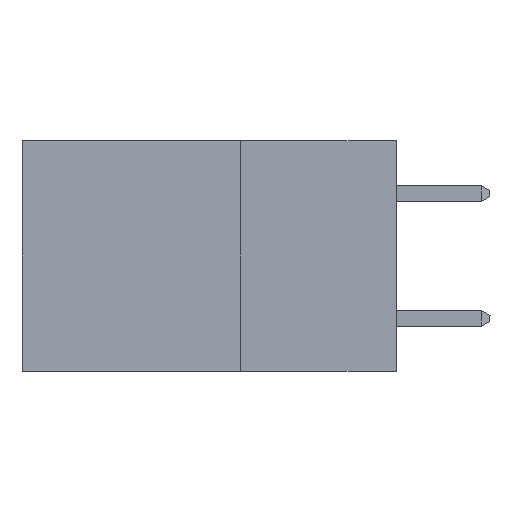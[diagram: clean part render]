
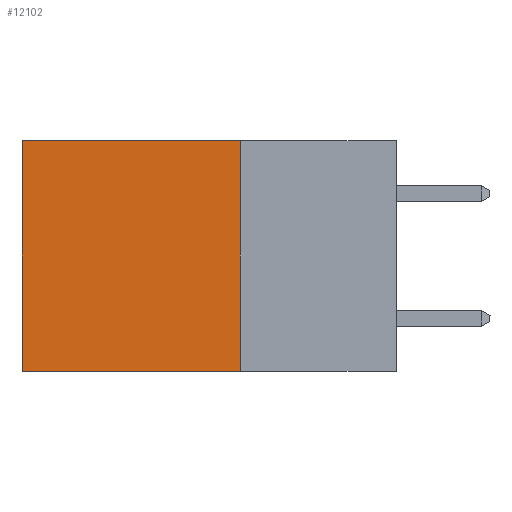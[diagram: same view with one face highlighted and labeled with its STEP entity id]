
A CAD part, left-side view. The second image highlights one B-rep face of the part: STEP entity #12102.
In plain terms, the highlighted planar face has unit normal (-1, 0, 0).
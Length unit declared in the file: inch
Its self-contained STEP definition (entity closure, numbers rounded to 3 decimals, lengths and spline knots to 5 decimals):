
#107 = ORIENTED_EDGE ( 'NONE', *, *, #2222, .F. ) ;
#369 = CARTESIAN_POINT ( 'NONE',  ( 0.298, 0.25, 0. ) ) ;
#804 = VECTOR ( 'NONE', #8576, 39.37008 ) ;
#810 = ORIENTED_EDGE ( 'NONE', *, *, #1115, .F. ) ;
#884 = LINE ( 'NONE', #2902, #11314 ) ;
#1019 = DIRECTION ( 'NONE',  ( 0., 1., 0. ) ) ;
#1040 = FACE_OUTER_BOUND ( 'NONE', #1140, .T. ) ;
#1115 = EDGE_CURVE ( 'NONE', #3930, #13056, #884, .T. ) ;
#1140 = EDGE_LOOP ( 'NONE', ( #1983, #810, #107, #2429 ) ) ;
#1565 = VERTEX_POINT ( 'NONE', #3058 ) ;
#1983 = ORIENTED_EDGE ( 'NONE', *, *, #12926, .T. ) ;
#2112 = VECTOR ( 'NONE', #3711, 39.37008 ) ;
#2222 = EDGE_CURVE ( 'NONE', #1565, #3930, #12969, .T. ) ;
#2429 = ORIENTED_EDGE ( 'NONE', *, *, #7800, .T. ) ;
#2902 = CARTESIAN_POINT ( 'NONE',  ( 0.298, 0.25, -0.37 ) ) ;
#3058 = CARTESIAN_POINT ( 'NONE',  ( 0.298, 0.25, 0. ) ) ;
#3431 = PLANE ( 'NONE',  #4601 ) ;
#3484 = VECTOR ( 'NONE', #5892, 39.37008 ) ;
#3711 = DIRECTION ( 'NONE',  ( 0., 0., -1. ) ) ;
#3930 = VERTEX_POINT ( 'NONE', #4106 ) ;
#4106 = CARTESIAN_POINT ( 'NONE',  ( 0.298, 0.25, -0.37 ) ) ;
#4601 = AXIS2_PLACEMENT_3D ( 'NONE', #8439, #10559, #10511 ) ;
#4845 = CARTESIAN_POINT ( 'NONE',  ( 0.298, 0.6, 0. ) ) ;
#5892 = DIRECTION ( 'NONE',  ( 0., 1., 0. ) ) ;
#5973 = CARTESIAN_POINT ( 'NONE',  ( 0.298, 0.25, 0. ) ) ;
#6321 = CARTESIAN_POINT ( 'NONE',  ( 0.298, 0.6, -0.37 ) ) ;
#7796 = CARTESIAN_POINT ( 'NONE',  ( 0.298, 0.6, 0. ) ) ;
#7800 = EDGE_CURVE ( 'NONE', #1565, #10502, #10627, .T. ) ;
#8439 = CARTESIAN_POINT ( 'NONE',  ( 0.298, 0.25, 0. ) ) ;
#8576 = DIRECTION ( 'NONE',  ( 0., 0., -1. ) ) ;
#8921 = LINE ( 'NONE', #4845, #2112 ) ;
#10502 = VERTEX_POINT ( 'NONE', #7796 ) ;
#10511 = DIRECTION ( 'NONE',  ( 0., 0., -1. ) ) ;
#10559 = DIRECTION ( 'NONE',  ( 1., 0., 0. ) ) ;
#10627 = LINE ( 'NONE', #5973, #3484 ) ;
#11314 = VECTOR ( 'NONE', #1019, 39.37008 ) ;
#12102 = ADVANCED_FACE ( 'NONE', ( #1040 ), #3431, .F. ) ;
#12926 = EDGE_CURVE ( 'NONE', #10502, #13056, #8921, .T. ) ;
#12969 = LINE ( 'NONE', #369, #804 ) ;
#13056 = VERTEX_POINT ( 'NONE', #6321 ) ;
